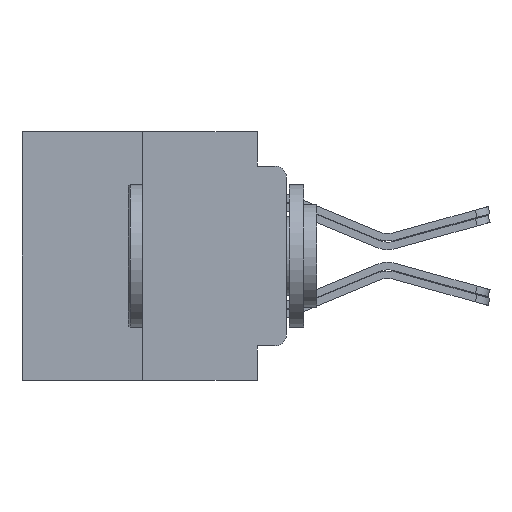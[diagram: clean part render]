
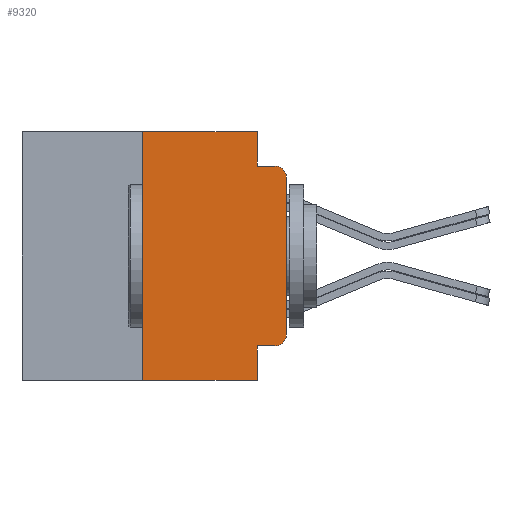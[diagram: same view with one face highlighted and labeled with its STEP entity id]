
A CAD part, left-side view. The second image highlights one B-rep face of the part: STEP entity #9320.
In plain terms, the highlighted planar face has unit normal (-1, 0, 0).
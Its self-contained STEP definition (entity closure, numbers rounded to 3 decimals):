
#127 = CIRCLE ( 'NONE', #7392, 0.508 ) ;
#248 = VECTOR ( 'NONE', #7673, 1000. ) ;
#316 = VECTOR ( 'NONE', #16146, 1000. ) ;
#2402 = ORIENTED_EDGE ( 'NONE', *, *, #8691, .T. ) ;
#2566 = CARTESIAN_POINT ( 'NONE',  ( -75.603, 1.295, -5.486 ) ) ;
#2695 = CARTESIAN_POINT ( 'NONE',  ( -75.603, 1.295, 3.975 ) ) ;
#3003 = VERTEX_POINT ( 'NONE', #18396 ) ;
#3112 = CARTESIAN_POINT ( 'NONE',  ( -75.603, 1.295, 5.486 ) ) ;
#4890 = VERTEX_POINT ( 'NONE', #3112 ) ;
#5284 = ORIENTED_EDGE ( 'NONE', *, *, #22127, .F. ) ;
#5336 = ORIENTED_EDGE ( 'NONE', *, *, #24047, .T. ) ;
#5558 = CARTESIAN_POINT ( 'NONE',  ( -75.603, 1.295, 3.975 ) ) ;
#5589 = AXIS2_PLACEMENT_3D ( 'NONE', #20045, #15180, #6245 ) ;
#5658 = DIRECTION ( 'NONE',  ( -1., 0., 0. ) ) ;
#6214 = VERTEX_POINT ( 'NONE', #2566 ) ;
#6245 = DIRECTION ( 'NONE',  ( 0., 0., -1. ) ) ;
#6392 = DIRECTION ( 'NONE',  ( 0., -1., 0. ) ) ;
#6481 = VECTOR ( 'NONE', #11738, 1000. ) ;
#6515 = LINE ( 'NONE', #22132, #22642 ) ;
#7392 = AXIS2_PLACEMENT_3D ( 'NONE', #28665, #5658, #23805 ) ;
#7673 = DIRECTION ( 'NONE',  ( 0., 0., 1. ) ) ;
#8003 = VECTOR ( 'NONE', #23327, 1000. ) ;
#8175 = EDGE_CURVE ( 'NONE', #21805, #4890, #28785, .T. ) ;
#8244 = EDGE_CURVE ( 'NONE', #4890, #20479, #6515, .T. ) ;
#8691 = EDGE_CURVE ( 'NONE', #18091, #23149, #11498, .T. ) ;
#8780 = EDGE_CURVE ( 'NONE', #18091, #6214, #26568, .T. ) ;
#8934 = DIRECTION ( 'NONE',  ( 0., 0., -1. ) ) ;
#9069 = EDGE_LOOP ( 'NONE', ( #2402, #21713, #23733, #15446, #5284, #15255, #14182, #12075, #5336, #27762 ) ) ;
#9229 = CIRCLE ( 'NONE', #14496, 0.508 ) ;
#9320 = ADVANCED_FACE ( 'NONE', ( #9692 ), #15476, .F. ) ;
#9577 = EDGE_CURVE ( 'NONE', #23620, #21805, #13981, .T. ) ;
#9692 = FACE_OUTER_BOUND ( 'NONE', #9069, .T. ) ;
#11498 = LINE ( 'NONE', #14742, #18671 ) ;
#11551 = CARTESIAN_POINT ( 'NONE',  ( -75.603, 0.508, -3.467 ) ) ;
#11738 = DIRECTION ( 'NONE',  ( 0., 0., -1. ) ) ;
#11779 = LINE ( 'NONE', #19246, #248 ) ;
#11839 = CARTESIAN_POINT ( 'NONE',  ( -75.603, 11.684, -5.486 ) ) ;
#11926 = EDGE_CURVE ( 'NONE', #25039, #17991, #11779, .T. ) ;
#12075 = ORIENTED_EDGE ( 'NONE', *, *, #9577, .F. ) ;
#12395 = EDGE_CURVE ( 'NONE', #23149, #25039, #9229, .T. ) ;
#12870 = CARTESIAN_POINT ( 'NONE',  ( -75.603, 6.35, -5.486 ) ) ;
#13103 = CARTESIAN_POINT ( 'NONE',  ( -75.603, 0.508, -3.975 ) ) ;
#13856 = CARTESIAN_POINT ( 'NONE',  ( -75.603, 6.35, -5.486 ) ) ;
#13981 = LINE ( 'NONE', #13856, #316 ) ;
#14182 = ORIENTED_EDGE ( 'NONE', *, *, #8175, .F. ) ;
#14496 = AXIS2_PLACEMENT_3D ( 'NONE', #11551, #23151, #18628 ) ;
#14636 = DIRECTION ( 'NONE',  ( 0., -1., 0. ) ) ;
#14742 = CARTESIAN_POINT ( 'NONE',  ( -75.603, 1.295, -3.975 ) ) ;
#15180 = DIRECTION ( 'NONE',  ( 1., 0., 0. ) ) ;
#15255 = ORIENTED_EDGE ( 'NONE', *, *, #8244, .F. ) ;
#15446 = ORIENTED_EDGE ( 'NONE', *, *, #20541, .T. ) ;
#15476 = PLANE ( 'NONE',  #5589 ) ;
#15798 = VECTOR ( 'NONE', #14636, 1000. ) ;
#16146 = DIRECTION ( 'NONE',  ( 0., 0., 1. ) ) ;
#16424 = CARTESIAN_POINT ( 'NONE',  ( -75.603, 1.295, 0. ) ) ;
#16447 = CARTESIAN_POINT ( 'NONE',  ( -75.603, 0., 3.467 ) ) ;
#17991 = VERTEX_POINT ( 'NONE', #16447 ) ;
#18091 = VERTEX_POINT ( 'NONE', #23840 ) ;
#18396 = CARTESIAN_POINT ( 'NONE',  ( -75.603, 0.508, 3.975 ) ) ;
#18628 = DIRECTION ( 'NONE',  ( 0., 0., -1. ) ) ;
#18671 = VECTOR ( 'NONE', #6392, 1000. ) ;
#19246 = CARTESIAN_POINT ( 'NONE',  ( -75.603, 0., 5.486 ) ) ;
#20045 = CARTESIAN_POINT ( 'NONE',  ( -75.603, 11.684, 5.486 ) ) ;
#20051 = DIRECTION ( 'NONE',  ( 0., -1., 0. ) ) ;
#20479 = VERTEX_POINT ( 'NONE', #5558 ) ;
#20541 = EDGE_CURVE ( 'NONE', #17991, #3003, #127, .T. ) ;
#21552 = VECTOR ( 'NONE', #20051, 1000. ) ;
#21713 = ORIENTED_EDGE ( 'NONE', *, *, #12395, .T. ) ;
#21805 = VERTEX_POINT ( 'NONE', #26213 ) ;
#22127 = EDGE_CURVE ( 'NONE', #20479, #3003, #23368, .T. ) ;
#22132 = CARTESIAN_POINT ( 'NONE',  ( -75.603, 1.295, 0. ) ) ;
#22642 = VECTOR ( 'NONE', #8934, 1000. ) ;
#23149 = VERTEX_POINT ( 'NONE', #13103 ) ;
#23151 = DIRECTION ( 'NONE',  ( -1., 0., 0. ) ) ;
#23327 = DIRECTION ( 'NONE',  ( 0., -1., 0. ) ) ;
#23368 = LINE ( 'NONE', #2695, #8003 ) ;
#23620 = VERTEX_POINT ( 'NONE', #12870 ) ;
#23733 = ORIENTED_EDGE ( 'NONE', *, *, #11926, .T. ) ;
#23805 = DIRECTION ( 'NONE',  ( 0., 0., -1. ) ) ;
#23840 = CARTESIAN_POINT ( 'NONE',  ( -75.603, 1.295, -3.975 ) ) ;
#24047 = EDGE_CURVE ( 'NONE', #23620, #6214, #25464, .T. ) ;
#25039 = VERTEX_POINT ( 'NONE', #25236 ) ;
#25236 = CARTESIAN_POINT ( 'NONE',  ( -75.603, 0., -3.467 ) ) ;
#25464 = LINE ( 'NONE', #11839, #15798 ) ;
#26213 = CARTESIAN_POINT ( 'NONE',  ( -75.603, 6.35, 5.486 ) ) ;
#26326 = CARTESIAN_POINT ( 'NONE',  ( -75.603, 11.684, 5.486 ) ) ;
#26568 = LINE ( 'NONE', #16424, #6481 ) ;
#27762 = ORIENTED_EDGE ( 'NONE', *, *, #8780, .F. ) ;
#28665 = CARTESIAN_POINT ( 'NONE',  ( -75.603, 0.508, 3.467 ) ) ;
#28785 = LINE ( 'NONE', #26326, #21552 ) ;
